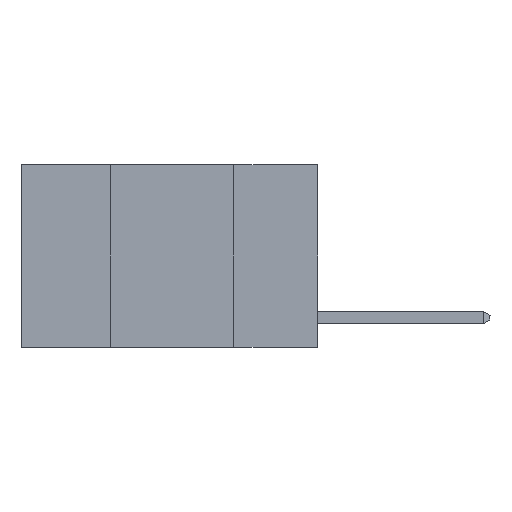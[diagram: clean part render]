
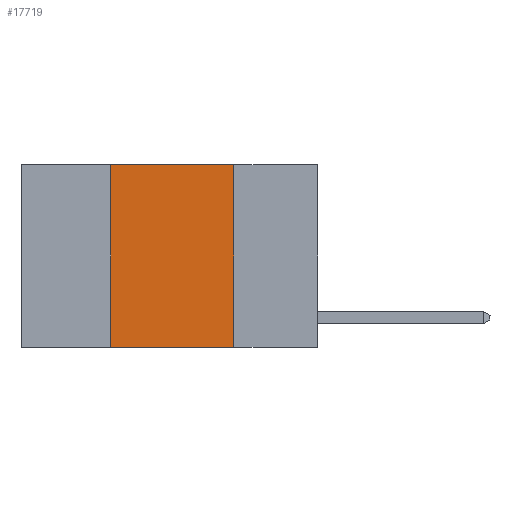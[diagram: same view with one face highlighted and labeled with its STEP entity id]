
A CAD part, left-side view. The second image highlights one B-rep face of the part: STEP entity #17719.
In plain terms, the highlighted planar face has unit normal (-1, 0, 0).
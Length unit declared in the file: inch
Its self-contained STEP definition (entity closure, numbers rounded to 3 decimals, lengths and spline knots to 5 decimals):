
#922 = DIRECTION ( 'NONE',  ( 0., 0., -1. ) ) ;
#1639 = VECTOR ( 'NONE', #8392, 39.37008 ) ;
#1982 = VECTOR ( 'NONE', #922, 39.37008 ) ;
#2073 = CARTESIAN_POINT ( 'NONE',  ( 0., 0.42, 0. ) ) ;
#2776 = CARTESIAN_POINT ( 'NONE',  ( 0., 0.17, -0.37 ) ) ;
#3070 = CARTESIAN_POINT ( 'NONE',  ( 0., 0.42, 0. ) ) ;
#3416 = EDGE_CURVE ( 'NONE', #13589, #11181, #13319, .T. ) ;
#3810 = ORIENTED_EDGE ( 'NONE', *, *, #14325, .F. ) ;
#5362 = ORIENTED_EDGE ( 'NONE', *, *, #12597, .F. ) ;
#5367 = PLANE ( 'NONE',  #13529 ) ;
#8103 = ORIENTED_EDGE ( 'NONE', *, *, #3416, .F. ) ;
#8392 = DIRECTION ( 'NONE',  ( 0., -1., 0. ) ) ;
#8518 = CARTESIAN_POINT ( 'NONE',  ( 0., 0.42, -0.37 ) ) ;
#8743 = DIRECTION ( 'NONE',  ( 0., 0., -1. ) ) ;
#9335 = VECTOR ( 'NONE', #9856, 39.37008 ) ;
#9856 = DIRECTION ( 'NONE',  ( 0., -1., 0. ) ) ;
#10100 = CARTESIAN_POINT ( 'NONE',  ( 0., 0.17, 0. ) ) ;
#10394 = VERTEX_POINT ( 'NONE', #2776 ) ;
#10488 = VERTEX_POINT ( 'NONE', #8518 ) ;
#11181 = VERTEX_POINT ( 'NONE', #10100 ) ;
#11680 = FACE_OUTER_BOUND ( 'NONE', #20793, .T. ) ;
#12128 = EDGE_CURVE ( 'NONE', #10488, #10394, #12533, .T. ) ;
#12533 = LINE ( 'NONE', #21945, #1639 ) ;
#12597 = EDGE_CURVE ( 'NONE', #10488, #13589, #21536, .T. ) ;
#13319 = LINE ( 'NONE', #20095, #9335 ) ;
#13529 = AXIS2_PLACEMENT_3D ( 'NONE', #13855, #17469, #8743 ) ;
#13589 = VERTEX_POINT ( 'NONE', #2073 ) ;
#13855 = CARTESIAN_POINT ( 'NONE',  ( 0., 0.6, 0. ) ) ;
#14325 = EDGE_CURVE ( 'NONE', #11181, #10394, #15552, .T. ) ;
#15552 = LINE ( 'NONE', #16340, #1982 ) ;
#16340 = CARTESIAN_POINT ( 'NONE',  ( 0., 0.17, 0. ) ) ;
#17469 = DIRECTION ( 'NONE',  ( 1., 0., 0. ) ) ;
#17719 = ADVANCED_FACE ( 'NONE', ( #11680 ), #5367, .F. ) ;
#17873 = ORIENTED_EDGE ( 'NONE', *, *, #12128, .T. ) ;
#18590 = VECTOR ( 'NONE', #20215, 39.37008 ) ;
#20095 = CARTESIAN_POINT ( 'NONE',  ( 0., 0.6, 0. ) ) ;
#20215 = DIRECTION ( 'NONE',  ( 0., 0., 1. ) ) ;
#20793 = EDGE_LOOP ( 'NONE', ( #3810, #8103, #5362, #17873 ) ) ;
#21536 = LINE ( 'NONE', #3070, #18590 ) ;
#21945 = CARTESIAN_POINT ( 'NONE',  ( 0., 0.6, -0.37 ) ) ;
